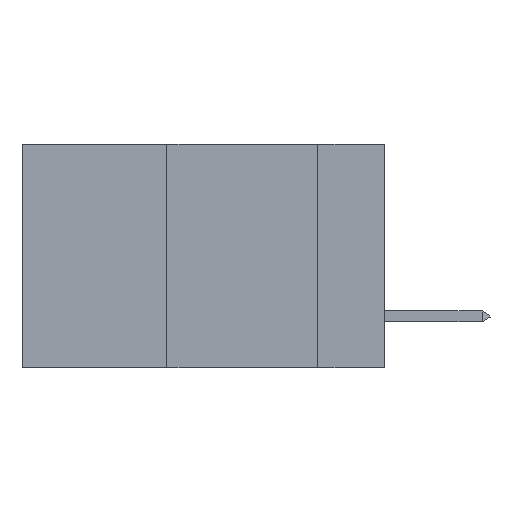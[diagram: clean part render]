
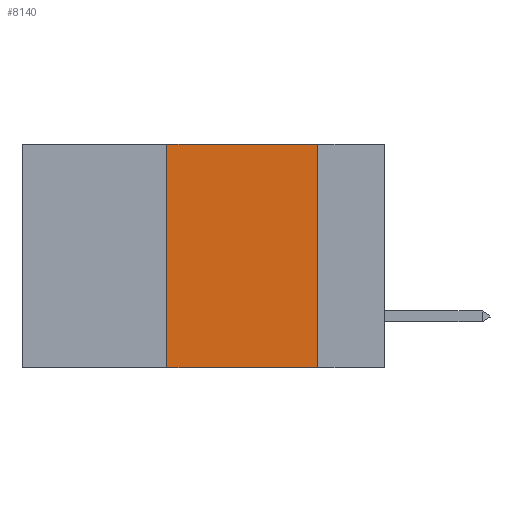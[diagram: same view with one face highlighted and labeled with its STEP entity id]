
A CAD part, left-side view. The second image highlights one B-rep face of the part: STEP entity #8140.
In plain terms, the highlighted planar face has unit normal (-1, 0, 0).
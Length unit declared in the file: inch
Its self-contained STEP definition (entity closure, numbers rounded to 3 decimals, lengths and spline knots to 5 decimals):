
#282 = VERTEX_POINT ( 'NONE', #29007 ) ;
#595 = ORIENTED_EDGE ( 'NONE', *, *, #11025, .F. ) ;
#789 = CARTESIAN_POINT ( 'NONE',  ( 0., 0.36, 0. ) ) ;
#3511 = VECTOR ( 'NONE', #14140, 39.37008 ) ;
#4793 = EDGE_CURVE ( 'NONE', #14077, #17159, #33579, .T. ) ;
#7308 = DIRECTION ( 'NONE',  ( 0., -1., 0. ) ) ;
#8140 = ADVANCED_FACE ( 'NONE', ( #16389 ), #44693, .F. ) ;
#8516 = ORIENTED_EDGE ( 'NONE', *, *, #23665, .F. ) ;
#9477 = VECTOR ( 'NONE', #7308, 39.37008 ) ;
#11025 = EDGE_CURVE ( 'NONE', #36302, #14077, #42937, .T. ) ;
#12572 = DIRECTION ( 'NONE',  ( 1., 0., 0. ) ) ;
#13880 = AXIS2_PLACEMENT_3D ( 'NONE', #23644, #12572, #34004 ) ;
#14077 = VERTEX_POINT ( 'NONE', #37564 ) ;
#14140 = DIRECTION ( 'NONE',  ( 0., -1., 0. ) ) ;
#14683 = CARTESIAN_POINT ( 'NONE',  ( 0., 0.6, -0.37 ) ) ;
#15484 = VECTOR ( 'NONE', #24320, 39.37008 ) ;
#16389 = FACE_OUTER_BOUND ( 'NONE', #21241, .T. ) ;
#17099 = CARTESIAN_POINT ( 'NONE',  ( 0., 0.36, 0. ) ) ;
#17159 = VERTEX_POINT ( 'NONE', #37309 ) ;
#20594 = ORIENTED_EDGE ( 'NONE', *, *, #4793, .F. ) ;
#21066 = LINE ( 'NONE', #14683, #3511 ) ;
#21241 = EDGE_LOOP ( 'NONE', ( #20594, #595, #8516, #29677 ) ) ;
#21687 = EDGE_CURVE ( 'NONE', #282, #17159, #21066, .T. ) ;
#23644 = CARTESIAN_POINT ( 'NONE',  ( 0., 0.6, 0. ) ) ;
#23665 = EDGE_CURVE ( 'NONE', #282, #36302, #44467, .T. ) ;
#24320 = DIRECTION ( 'NONE',  ( 0., 0., -1. ) ) ;
#29007 = CARTESIAN_POINT ( 'NONE',  ( 0., 0.36, -0.37 ) ) ;
#29677 = ORIENTED_EDGE ( 'NONE', *, *, #21687, .T. ) ;
#33579 = LINE ( 'NONE', #45388, #15484 ) ;
#34004 = DIRECTION ( 'NONE',  ( 0., 0., -1. ) ) ;
#36176 = CARTESIAN_POINT ( 'NONE',  ( 0., 0.6, 0. ) ) ;
#36302 = VERTEX_POINT ( 'NONE', #789 ) ;
#37309 = CARTESIAN_POINT ( 'NONE',  ( 0., 0.11, -0.37 ) ) ;
#37564 = CARTESIAN_POINT ( 'NONE',  ( 0., 0.11, 0. ) ) ;
#37910 = VECTOR ( 'NONE', #44071, 39.37008 ) ;
#42937 = LINE ( 'NONE', #36176, #9477 ) ;
#44071 = DIRECTION ( 'NONE',  ( 0., 0., 1. ) ) ;
#44467 = LINE ( 'NONE', #17099, #37910 ) ;
#44693 = PLANE ( 'NONE',  #13880 ) ;
#45388 = CARTESIAN_POINT ( 'NONE',  ( 0., 0.11, 0. ) ) ;
